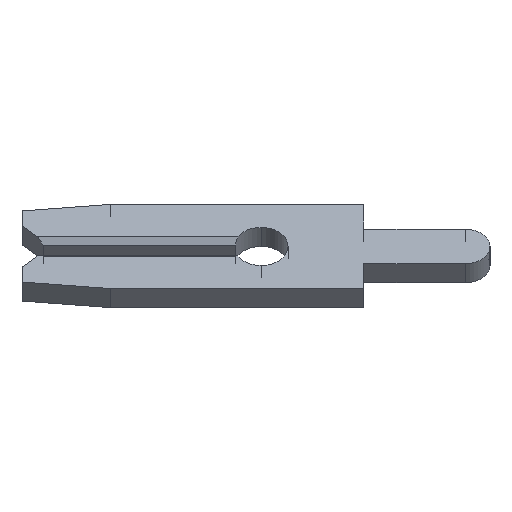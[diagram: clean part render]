
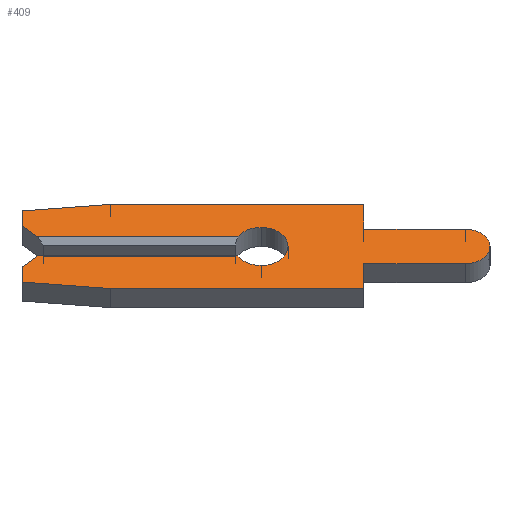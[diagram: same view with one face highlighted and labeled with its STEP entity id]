
A CAD part, left-side view. The second image highlights one B-rep face of the part: STEP entity #409.
In plain terms, the highlighted face is planar.
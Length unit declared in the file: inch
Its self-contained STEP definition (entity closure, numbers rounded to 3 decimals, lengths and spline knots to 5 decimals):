
#2 = EDGE_CURVE ( 'NONE', #1557, #394, #156, .T. ) ;
#4 = VERTEX_POINT ( 'NONE', #181 ) ;
#19 = ORIENTED_EDGE ( 'NONE', *, *, #1737, .T. ) ;
#20 = ORIENTED_EDGE ( 'NONE', *, *, #333, .F. ) ;
#28 = DIRECTION ( 'NONE',  ( 0., 1., 0. ) ) ;
#57 = DIRECTION ( 'NONE',  ( 0., 0., -1. ) ) ;
#70 = DIRECTION ( 'NONE',  ( 0., 0., -1. ) ) ;
#85 = ORIENTED_EDGE ( 'NONE', *, *, #1405, .F. ) ;
#88 = VECTOR ( 'NONE', #327, 39.37008 ) ;
#92 = DIRECTION ( 'NONE',  ( 0., 0., -1. ) ) ;
#96 = EDGE_CURVE ( 'NONE', #1112, #726, #1384, .T. ) ;
#111 = EDGE_CURVE ( 'NONE', #207, #894, #320, .T. ) ;
#142 = CARTESIAN_POINT ( 'NONE',  ( -0.013, 0., 0. ) ) ;
#156 = LINE ( 'NONE', #639, #1599 ) ;
#160 = CARTESIAN_POINT ( 'NONE',  ( -0.013, -0.099, -0.0235 ) ) ;
#181 = CARTESIAN_POINT ( 'NONE',  ( -0.013, 0., -0.026 ) ) ;
#207 = VERTEX_POINT ( 'NONE', #1538 ) ;
#208 = CARTESIAN_POINT ( 'NONE',  ( -0.013, 0.146, 0.0575 ) ) ;
#214 = PLANE ( 'NONE',  #1732 ) ;
#221 = DIRECTION ( 'NONE',  ( 0., -1., 0. ) ) ;
#223 = CARTESIAN_POINT ( 'NONE',  ( -0.013, -0.099, 0.0235 ) ) ;
#232 = VERTEX_POINT ( 'NONE', #1409 ) ;
#254 = DIRECTION ( 'NONE',  ( 0., 0.995, 0.105 ) ) ;
#255 = ORIENTED_EDGE ( 'NONE', *, *, #1152, .F. ) ;
#273 = CARTESIAN_POINT ( 'NONE',  ( -0.013, 0.231, 0.028 ) ) ;
#312 = VECTOR ( 'NONE', #416, 39.37008 ) ;
#320 = LINE ( 'NONE', #1227, #910 ) ;
#321 = VECTOR ( 'NONE', #28, 39.37008 ) ;
#327 = DIRECTION ( 'NONE',  ( 0., 1., 0. ) ) ;
#333 = EDGE_CURVE ( 'NONE', #1192, #1063, #630, .T. ) ;
#343 = CARTESIAN_POINT ( 'NONE',  ( -0.013, 0., 0. ) ) ;
#350 = DIRECTION ( 'NONE',  ( 0., 0., 1. ) ) ;
#355 = CARTESIAN_POINT ( 'NONE',  ( -0.013, -0.1975, -0.0235 ) ) ;
#365 = ORIENTED_EDGE ( 'NONE', *, *, #1325, .F. ) ;
#380 = VECTOR ( 'NONE', #1869, 39.37008 ) ;
#386 = VERTEX_POINT ( 'NONE', #645 ) ;
#394 = VERTEX_POINT ( 'NONE', #223 ) ;
#408 = LINE ( 'NONE', #953, #380 ) ;
#409 = ADVANCED_FACE ( 'NONE', ( #1356 ), #214, .F. ) ;
#416 = DIRECTION ( 'NONE',  ( 0., 0., 1. ) ) ;
#420 = LINE ( 'NONE', #1535, #1422 ) ;
#432 = EDGE_CURVE ( 'NONE', #799, #531, #1502, .T. ) ;
#439 = CARTESIAN_POINT ( 'NONE',  ( -0.013, 0.02252, -0.013 ) ) ;
#482 = CARTESIAN_POINT ( 'NONE',  ( -0.013, -0.1975, 0. ) ) ;
#524 = DIRECTION ( 'NONE',  ( 0., -1., 0. ) ) ;
#529 = DIRECTION ( 'NONE',  ( 1., 0., 0. ) ) ;
#531 = VERTEX_POINT ( 'NONE', #208 ) ;
#535 = CARTESIAN_POINT ( 'NONE',  ( -0.013, 0., 0. ) ) ;
#548 = EDGE_CURVE ( 'NONE', #1705, #915, #1579, .T. ) ;
#549 = CARTESIAN_POINT ( 'NONE',  ( -0.013, 0.146, -0.0575 ) ) ;
#561 = DIRECTION ( 'NONE',  ( -1., 0., 0. ) ) ;
#568 = EDGE_CURVE ( 'NONE', #232, #898, #685, .T. ) ;
#572 = ORIENTED_EDGE ( 'NONE', *, *, #111, .F. ) ;
#573 = CARTESIAN_POINT ( 'NONE',  ( -0.013, 0.231, 0.028 ) ) ;
#594 = ORIENTED_EDGE ( 'NONE', *, *, #1870, .F. ) ;
#630 = LINE ( 'NONE', #1090, #1144 ) ;
#631 = DIRECTION ( 'NONE',  ( 0., 0., -1. ) ) ;
#634 = CIRCLE ( 'NONE', #1660, 0.026 ) ;
#639 = CARTESIAN_POINT ( 'NONE',  ( -0.013, -0.099, 0.0575 ) ) ;
#645 = CARTESIAN_POINT ( 'NONE',  ( -0.013, -0.099, -0.0235 ) ) ;
#653 = CARTESIAN_POINT ( 'NONE',  ( -0.013, -0.1975, 0.0235 ) ) ;
#670 = CARTESIAN_POINT ( 'NONE',  ( -0.013, -0.099, 0.0575 ) ) ;
#685 = CIRCLE ( 'NONE', #914, 0.026 ) ;
#696 = LINE ( 'NONE', #273, #312 ) ;
#699 = LINE ( 'NONE', #1690, #1598 ) ;
#700 = ORIENTED_EDGE ( 'NONE', *, *, #2, .F. ) ;
#702 = LINE ( 'NONE', #160, #321 ) ;
#726 = VERTEX_POINT ( 'NONE', #549 ) ;
#736 = VECTOR ( 'NONE', #827, 39.37008 ) ;
#757 = EDGE_CURVE ( 'NONE', #726, #207, #817, .T. ) ;
#775 = DIRECTION ( 'NONE',  ( -1., 0., 0. ) ) ;
#799 = VERTEX_POINT ( 'NONE', #1611 ) ;
#805 = AXIS2_PLACEMENT_3D ( 'NONE', #482, #1519, #1796 ) ;
#813 = CARTESIAN_POINT ( 'NONE',  ( -0.013, 0.231, 0.013 ) ) ;
#817 = LINE ( 'NONE', #1605, #1284 ) ;
#821 = ORIENTED_EDGE ( 'NONE', *, *, #432, .F. ) ;
#827 = DIRECTION ( 'NONE',  ( 0., 0.707, 0.707 ) ) ;
#831 = DIRECTION ( 'NONE',  ( 0., -1., 0. ) ) ;
#839 = CARTESIAN_POINT ( 'NONE',  ( -0.013, -0.099, 0.0235 ) ) ;
#851 = ORIENTED_EDGE ( 'NONE', *, *, #548, .F. ) ;
#893 = CARTESIAN_POINT ( 'NONE',  ( -0.013, 0.216, -0.013 ) ) ;
#894 = VERTEX_POINT ( 'NONE', #1012 ) ;
#898 = VERTEX_POINT ( 'NONE', #1150 ) ;
#910 = VECTOR ( 'NONE', #350, 39.37008 ) ;
#914 = AXIS2_PLACEMENT_3D ( 'NONE', #535, #561, #92 ) ;
#915 = VERTEX_POINT ( 'NONE', #573 ) ;
#942 = ORIENTED_EDGE ( 'NONE', *, *, #1055, .F. ) ;
#953 = CARTESIAN_POINT ( 'NONE',  ( -0.013, 0.2105, -0.0075 ) ) ;
#966 = EDGE_LOOP ( 'NONE', ( #19, #1751, #942, #365, #20, #1474, #572, #1747, #1700, #1724, #1067, #255, #594, #700, #85, #821, #1157, #851 ) ) ;
#1004 = DIRECTION ( 'NONE',  ( 0., 0., -1. ) ) ;
#1007 = VECTOR ( 'NONE', #1864, 39.37008 ) ;
#1012 = CARTESIAN_POINT ( 'NONE',  ( -0.013, 0.231, -0.028 ) ) ;
#1031 = VERTEX_POINT ( 'NONE', #355 ) ;
#1040 = LINE ( 'NONE', #813, #1183 ) ;
#1055 = EDGE_CURVE ( 'NONE', #4, #232, #1478, .T. ) ;
#1063 = VERTEX_POINT ( 'NONE', #439 ) ;
#1067 = ORIENTED_EDGE ( 'NONE', *, *, #1095, .F. ) ;
#1087 = DIRECTION ( 'NONE',  ( 0., -1., 0. ) ) ;
#1090 = CARTESIAN_POINT ( 'NONE',  ( -0.013, 0., -0.013 ) ) ;
#1092 = CARTESIAN_POINT ( 'NONE',  ( -0.013, 0.216, 0.013 ) ) ;
#1095 = EDGE_CURVE ( 'NONE', #1031, #386, #702, .T. ) ;
#1109 = AXIS2_PLACEMENT_3D ( 'NONE', #142, #1174, #1004 ) ;
#1112 = VERTEX_POINT ( 'NONE', #1181 ) ;
#1137 = VECTOR ( 'NONE', #831, 39.37008 ) ;
#1144 = VECTOR ( 'NONE', #524, 39.37008 ) ;
#1150 = CARTESIAN_POINT ( 'NONE',  ( -0.013, 0.02252, 0.013 ) ) ;
#1152 = EDGE_CURVE ( 'NONE', #1386, #1031, #1440, .T. ) ;
#1157 = ORIENTED_EDGE ( 'NONE', *, *, #1845, .F. ) ;
#1174 = DIRECTION ( 'NONE',  ( -1., 0., 0. ) ) ;
#1181 = CARTESIAN_POINT ( 'NONE',  ( -0.013, -0.099, -0.0575 ) ) ;
#1183 = VECTOR ( 'NONE', #221, 39.37008 ) ;
#1192 = VERTEX_POINT ( 'NONE', #893 ) ;
#1227 = CARTESIAN_POINT ( 'NONE',  ( -0.013, 0.231, -0.028 ) ) ;
#1239 = DIRECTION ( 'NONE',  ( 0., 0., -1. ) ) ;
#1284 = VECTOR ( 'NONE', #254, 39.37008 ) ;
#1325 = EDGE_CURVE ( 'NONE', #1063, #4, #634, .T. ) ;
#1356 = FACE_OUTER_BOUND ( 'NONE', #966, .T. ) ;
#1384 = LINE ( 'NONE', #1835, #88 ) ;
#1386 = VERTEX_POINT ( 'NONE', #653 ) ;
#1405 = EDGE_CURVE ( 'NONE', #531, #1557, #699, .T. ) ;
#1409 = CARTESIAN_POINT ( 'NONE',  ( -0.013, 0., 0.026 ) ) ;
#1422 = VECTOR ( 'NONE', #57, 39.37008 ) ;
#1433 = CARTESIAN_POINT ( 'NONE',  ( -0.013, 0.2105, 0.0075 ) ) ;
#1440 = CIRCLE ( 'NONE', #805, 0.0235 ) ;
#1474 = ORIENTED_EDGE ( 'NONE', *, *, #1777, .F. ) ;
#1478 = CIRCLE ( 'NONE', #1109, 0.026 ) ;
#1498 = EDGE_CURVE ( 'NONE', #386, #1112, #420, .T. ) ;
#1502 = LINE ( 'NONE', #1555, #1007 ) ;
#1519 = DIRECTION ( 'NONE',  ( 1., 0., 0. ) ) ;
#1535 = CARTESIAN_POINT ( 'NONE',  ( -0.013, -0.099, -0.0575 ) ) ;
#1538 = CARTESIAN_POINT ( 'NONE',  ( -0.013, 0.231, -0.04857 ) ) ;
#1555 = CARTESIAN_POINT ( 'NONE',  ( -0.013, 0.231, 0.04857 ) ) ;
#1557 = VERTEX_POINT ( 'NONE', #670 ) ;
#1579 = LINE ( 'NONE', #1433, #736 ) ;
#1598 = VECTOR ( 'NONE', #1087, 39.37008 ) ;
#1599 = VECTOR ( 'NONE', #631, 39.37008 ) ;
#1605 = CARTESIAN_POINT ( 'NONE',  ( -0.013, 0.231, -0.04857 ) ) ;
#1611 = CARTESIAN_POINT ( 'NONE',  ( -0.013, 0.231, 0.04857 ) ) ;
#1660 = AXIS2_PLACEMENT_3D ( 'NONE', #343, #775, #1239 ) ;
#1690 = CARTESIAN_POINT ( 'NONE',  ( -0.013, 0.146, 0.0575 ) ) ;
#1700 = ORIENTED_EDGE ( 'NONE', *, *, #96, .F. ) ;
#1705 = VERTEX_POINT ( 'NONE', #1092 ) ;
#1724 = ORIENTED_EDGE ( 'NONE', *, *, #1498, .F. ) ;
#1732 = AXIS2_PLACEMENT_3D ( 'NONE', #1856, #529, #70 ) ;
#1737 = EDGE_CURVE ( 'NONE', #1705, #898, #1040, .T. ) ;
#1747 = ORIENTED_EDGE ( 'NONE', *, *, #757, .F. ) ;
#1751 = ORIENTED_EDGE ( 'NONE', *, *, #568, .F. ) ;
#1777 = EDGE_CURVE ( 'NONE', #894, #1192, #408, .T. ) ;
#1796 = DIRECTION ( 'NONE',  ( 0., 0., 1. ) ) ;
#1810 = LINE ( 'NONE', #839, #1137 ) ;
#1835 = CARTESIAN_POINT ( 'NONE',  ( -0.013, 0.146, -0.0575 ) ) ;
#1845 = EDGE_CURVE ( 'NONE', #915, #799, #696, .T. ) ;
#1856 = CARTESIAN_POINT ( 'NONE',  ( -0.013, 0., 0. ) ) ;
#1864 = DIRECTION ( 'NONE',  ( 0., -0.995, 0.105 ) ) ;
#1869 = DIRECTION ( 'NONE',  ( 0., -0.707, 0.707 ) ) ;
#1870 = EDGE_CURVE ( 'NONE', #394, #1386, #1810, .T. ) ;
